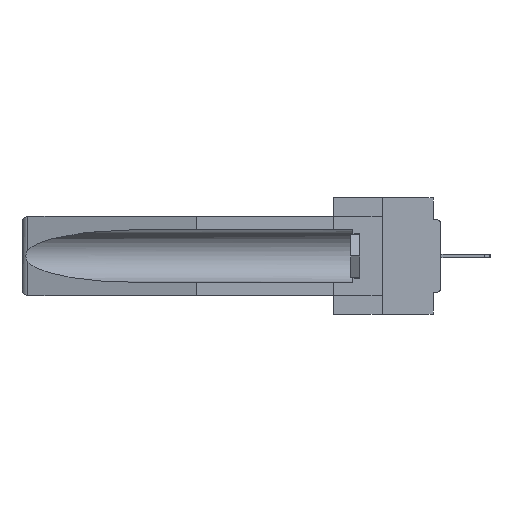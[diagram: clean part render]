
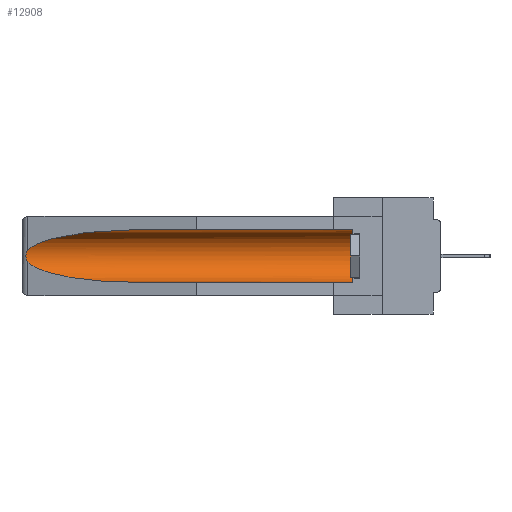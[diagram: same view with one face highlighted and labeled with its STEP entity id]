
A CAD part, left-side view. The second image highlights one B-rep face of the part: STEP entity #12908.
In plain terms, the highlighted cylindrical face has radius 2.857 mm (diameter 5.715 mm), a partial arc.
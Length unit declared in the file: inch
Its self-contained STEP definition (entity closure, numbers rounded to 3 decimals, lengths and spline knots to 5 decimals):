
#186 = ORIENTED_EDGE ( 'NONE', *, *, #11345, .T. ) ;
#2160 = VERTEX_POINT ( 'NONE', #15816 ) ;
#2426 = DIRECTION ( 'NONE',  ( 0., 0., 1. ) ) ;
#2510 = VERTEX_POINT ( 'NONE', #8108 ) ;
#2733 = EDGE_CURVE ( 'NONE', #16435, #7299, #29686, .T. ) ;
#3140 = B_SPLINE_CURVE_WITH_KNOTS ( 'NONE', 3,
 ( #19168, #16691, #21644, #6792, #24117, #9288, #26586, #11779, #29039, #14310 ),
 .UNSPECIFIED., .F., .F.,
 ( 4, 2, 2, 2, 4 ),
 ( 0., 0.00029, 0.00058, 0.00087, 0.00117 ),
 .UNSPECIFIED. ) ;
#5456 = EDGE_LOOP ( 'NONE', ( #8092, #16361, #186, #16264, #16651, #26436 ) ) ;
#5596 = CARTESIAN_POINT ( 'NONE',  ( 0.155, 1.07973, -0.059 ) ) ;
#5625 = CYLINDRICAL_SURFACE ( 'NONE', #8219, 0.1125 ) ;
#6202 = VERTEX_POINT ( 'NONE', #5596 ) ;
#6792 = CARTESIAN_POINT ( 'NONE',  ( 0.2673, 1.5327, -0.16383 ) ) ;
#7077 = DIRECTION ( 'NONE',  ( 0., 1., 0. ) ) ;
#7082 = DIRECTION ( 'NONE',  ( 0., 1., 0. ) ) ;
#7299 = VERTEX_POINT ( 'NONE', #11732 ) ;
#7390 = CARTESIAN_POINT ( 'NONE',  ( 0.155, -0.30754, -0.1715 ) ) ;
#8092 = ORIENTED_EDGE ( 'NONE', *, *, #12165, .T. ) ;
#8108 = CARTESIAN_POINT ( 'NONE',  ( 0.155, 1.07973, -0.284 ) ) ;
#8219 = AXIS2_PLACEMENT_3D ( 'NONE', #7390, #22115, #2426 ) ;
#8875 =( BOUNDED_CURVE ( )  B_SPLINE_CURVE ( 3, ( #14164, #28902, #31325, #16650 ),
 .UNSPECIFIED., .F., .T. ) 
 B_SPLINE_CURVE_WITH_KNOTS ( ( 4, 4 ),
 ( 0.1948, 1.5708 ),
 .UNSPECIFIED. ) 
 CURVE ( )  GEOMETRIC_REPRESENTATION_ITEM ( )  RATIONAL_B_SPLINE_CURVE ( ( 1., 0.848, 0.848, 1. ) ) 
 REPRESENTATION_ITEM ( '' )  );
#9288 = CARTESIAN_POINT ( 'NONE',  ( 0.2675, 1.53308, -0.17534 ) ) ;
#9987 = LINE ( 'NONE', #14589, #28155 ) ;
#10738 = EDGE_CURVE ( 'NONE', #2160, #30985, #3140, .T. ) ;
#11345 = EDGE_CURVE ( 'NONE', #30985, #2510, #8875, .T. ) ;
#11431 = CARTESIAN_POINT ( 'NONE',  ( 0.21114, 1.30732, -0.059 ) ) ;
#11732 = CARTESIAN_POINT ( 'NONE',  ( 0.155, 0.126, -0.059 ) ) ;
#11779 = CARTESIAN_POINT ( 'NONE',  ( 0.26655, 1.53094, -0.18657 ) ) ;
#12165 = EDGE_CURVE ( 'NONE', #6202, #2160, #20429, .T. ) ;
#12908 = ADVANCED_FACE ( 'NONE', ( #13019 ), #5625, .F. ) ;
#13019 = FACE_OUTER_BOUND ( 'NONE', #5456, .T. ) ;
#14067 = CARTESIAN_POINT ( 'NONE',  ( 0.25451, 1.48313, -0.09465 ) ) ;
#14164 = CARTESIAN_POINT ( 'NONE',  ( 0.26537, 1.52718, -0.19328 ) ) ;
#14310 = CARTESIAN_POINT ( 'NONE',  ( 0.26537, 1.52718, -0.19328 ) ) ;
#14589 = CARTESIAN_POINT ( 'NONE',  ( 0.155, -0.30754, -0.284 ) ) ;
#15281 = VECTOR ( 'NONE', #7077, 39.37008 ) ;
#15816 = CARTESIAN_POINT ( 'NONE',  ( 0.26537, 1.52718, -0.14972 ) ) ;
#16264 = ORIENTED_EDGE ( 'NONE', *, *, #17707, .F. ) ;
#16361 = ORIENTED_EDGE ( 'NONE', *, *, #10738, .T. ) ;
#16435 = VERTEX_POINT ( 'NONE', #17832 ) ;
#16650 = CARTESIAN_POINT ( 'NONE',  ( 0.155, 1.07973, -0.284 ) ) ;
#16651 = ORIENTED_EDGE ( 'NONE', *, *, #2733, .T. ) ;
#16691 = CARTESIAN_POINT ( 'NONE',  ( 0.26597, 1.52961, -0.15275 ) ) ;
#17707 = EDGE_CURVE ( 'NONE', #16435, #2510, #9987, .T. ) ;
#17832 = CARTESIAN_POINT ( 'NONE',  ( 0.155, 0.126, -0.284 ) ) ;
#18925 = CARTESIAN_POINT ( 'NONE',  ( 0.155, 1.07973, -0.059 ) ) ;
#19168 = CARTESIAN_POINT ( 'NONE',  ( 0.26537, 1.52718, -0.14972 ) ) ;
#20429 =( BOUNDED_CURVE ( )  B_SPLINE_CURVE ( 3, ( #18925, #11431, #14067, #31236 ),
 .UNSPECIFIED., .F., .F. ) 
 B_SPLINE_CURVE_WITH_KNOTS ( ( 4, 4 ),
 ( 4.71239, 6.08839 ),
 .UNSPECIFIED. ) 
 CURVE ( )  GEOMETRIC_REPRESENTATION_ITEM ( )  RATIONAL_B_SPLINE_CURVE ( ( 1., 0.848, 0.848, 1. ) ) 
 REPRESENTATION_ITEM ( '' )  );
#21644 = CARTESIAN_POINT ( 'NONE',  ( 0.26654, 1.53092, -0.15636 ) ) ;
#21827 = LINE ( 'NONE', #24404, #15281 ) ;
#22115 = DIRECTION ( 'NONE',  ( 0., 1., 0. ) ) ;
#22268 = AXIS2_PLACEMENT_3D ( 'NONE', #29242, #27735, #27699 ) ;
#24117 = CARTESIAN_POINT ( 'NONE',  ( 0.2675, 1.53308, -0.16763 ) ) ;
#24404 = CARTESIAN_POINT ( 'NONE',  ( 0.155, -0.30754, -0.059 ) ) ;
#26436 = ORIENTED_EDGE ( 'NONE', *, *, #29160, .T. ) ;
#26586 = CARTESIAN_POINT ( 'NONE',  ( 0.2673, 1.53269, -0.17917 ) ) ;
#27699 = DIRECTION ( 'NONE',  ( 0., 0., 1. ) ) ;
#27735 = DIRECTION ( 'NONE',  ( 0., -1., 0. ) ) ;
#28155 = VECTOR ( 'NONE', #7082, 39.37008 ) ;
#28902 = CARTESIAN_POINT ( 'NONE',  ( 0.25451, 1.48313, -0.24835 ) ) ;
#29039 = CARTESIAN_POINT ( 'NONE',  ( 0.26597, 1.5296, -0.19026 ) ) ;
#29160 = EDGE_CURVE ( 'NONE', #7299, #6202, #21827, .T. ) ;
#29242 = CARTESIAN_POINT ( 'NONE',  ( 0.155, 0.126, -0.1715 ) ) ;
#29409 = CARTESIAN_POINT ( 'NONE',  ( 0.26537, 1.52718, -0.19328 ) ) ;
#29686 = CIRCLE ( 'NONE', #22268, 0.1125 ) ;
#30985 = VERTEX_POINT ( 'NONE', #29409 ) ;
#31236 = CARTESIAN_POINT ( 'NONE',  ( 0.26537, 1.52718, -0.14972 ) ) ;
#31325 = CARTESIAN_POINT ( 'NONE',  ( 0.21114, 1.30732, -0.284 ) ) ;
